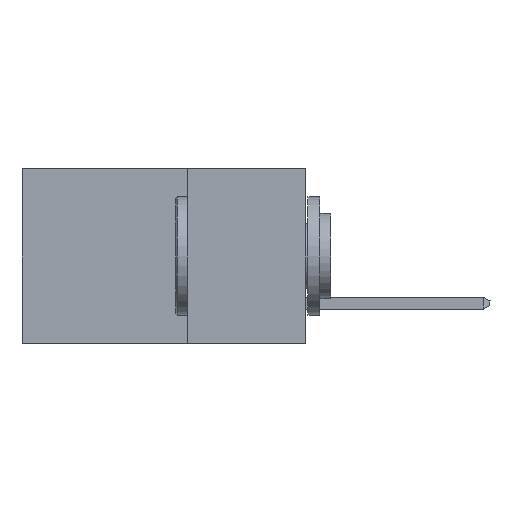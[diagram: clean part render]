
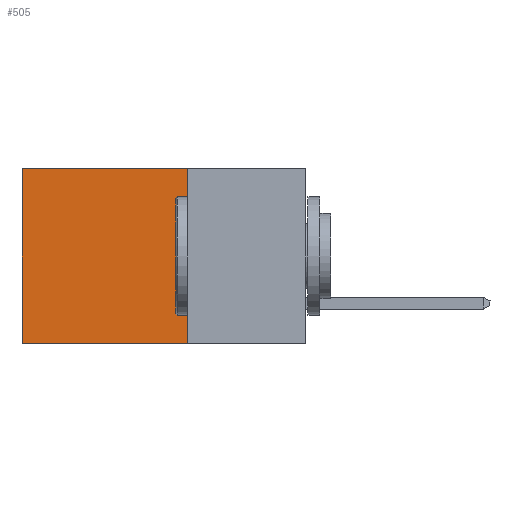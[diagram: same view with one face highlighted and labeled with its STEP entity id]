
A CAD part, left-side view. The second image highlights one B-rep face of the part: STEP entity #505.
In plain terms, the highlighted planar face has unit normal (-1, 0, 0).
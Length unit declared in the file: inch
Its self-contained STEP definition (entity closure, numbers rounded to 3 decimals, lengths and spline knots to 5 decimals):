
#425 = EDGE_CURVE ( 'NONE', #3864, #7919, #2727, .T. ) ;
#505 = ADVANCED_FACE ( 'NONE', ( #8536 ), #1018, .F. ) ;
#821 = LINE ( 'NONE', #2649, #12312 ) ;
#881 = DIRECTION ( 'NONE',  ( 0., 1., 0. ) ) ;
#1018 = PLANE ( 'NONE',  #5124 ) ;
#1179 = CARTESIAN_POINT ( 'NONE',  ( 0.2615, 0.6, 0. ) ) ;
#1531 = LINE ( 'NONE', #1591, #8972 ) ;
#1591 = CARTESIAN_POINT ( 'NONE',  ( 0.2615, 0.6, -0.37 ) ) ;
#2251 = LINE ( 'NONE', #7017, #9950 ) ;
#2649 = CARTESIAN_POINT ( 'NONE',  ( 0.2615, 0.25, -0.37 ) ) ;
#2727 = LINE ( 'NONE', #5783, #6108 ) ;
#2856 = ORIENTED_EDGE ( 'NONE', *, *, #425, .T. ) ;
#2876 = ORIENTED_EDGE ( 'NONE', *, *, #7476, .F. ) ;
#3864 = VERTEX_POINT ( 'NONE', #9076 ) ;
#4572 = CARTESIAN_POINT ( 'NONE',  ( 0.2615, 0.6, -0.37 ) ) ;
#4879 = DIRECTION ( 'NONE',  ( 0., 0., -1. ) ) ;
#5121 = ORIENTED_EDGE ( 'NONE', *, *, #11026, .T. ) ;
#5124 = AXIS2_PLACEMENT_3D ( 'NONE', #6776, #8478, #7594 ) ;
#5783 = CARTESIAN_POINT ( 'NONE',  ( 0.2615, 0.25, 0. ) ) ;
#6108 = VECTOR ( 'NONE', #12247, 39.37008 ) ;
#6293 = EDGE_LOOP ( 'NONE', ( #5121, #7032, #2876, #2856 ) ) ;
#6776 = CARTESIAN_POINT ( 'NONE',  ( 0.2615, 0.25, -0.37 ) ) ;
#7017 = CARTESIAN_POINT ( 'NONE',  ( 0.2615, 0.25, -0.37 ) ) ;
#7032 = ORIENTED_EDGE ( 'NONE', *, *, #7342, .F. ) ;
#7342 = EDGE_CURVE ( 'NONE', #12192, #10160, #821, .T. ) ;
#7476 = EDGE_CURVE ( 'NONE', #3864, #12192, #2251, .T. ) ;
#7594 = DIRECTION ( 'NONE',  ( 0., 0., -1. ) ) ;
#7919 = VERTEX_POINT ( 'NONE', #1179 ) ;
#8478 = DIRECTION ( 'NONE',  ( 1., 0., 0. ) ) ;
#8536 = FACE_OUTER_BOUND ( 'NONE', #6293, .T. ) ;
#8972 = VECTOR ( 'NONE', #9252, 39.37008 ) ;
#9076 = CARTESIAN_POINT ( 'NONE',  ( 0.2615, 0.25, 0. ) ) ;
#9252 = DIRECTION ( 'NONE',  ( 0., 0., -1. ) ) ;
#9950 = VECTOR ( 'NONE', #4879, 39.37008 ) ;
#10160 = VERTEX_POINT ( 'NONE', #4572 ) ;
#10953 = CARTESIAN_POINT ( 'NONE',  ( 0.2615, 0.25, -0.37 ) ) ;
#11026 = EDGE_CURVE ( 'NONE', #7919, #10160, #1531, .T. ) ;
#12192 = VERTEX_POINT ( 'NONE', #10953 ) ;
#12247 = DIRECTION ( 'NONE',  ( 0., 1., 0. ) ) ;
#12312 = VECTOR ( 'NONE', #881, 39.37008 ) ;
